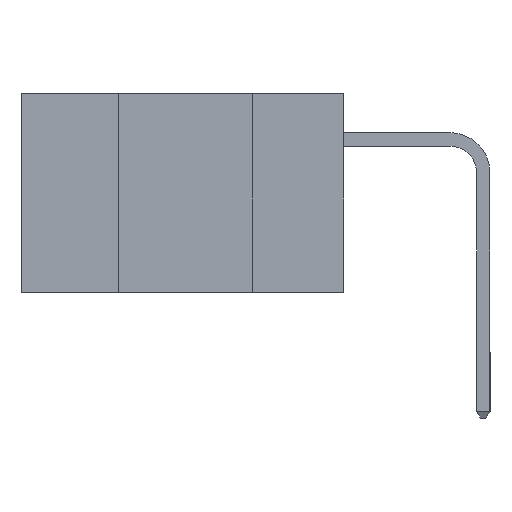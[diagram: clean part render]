
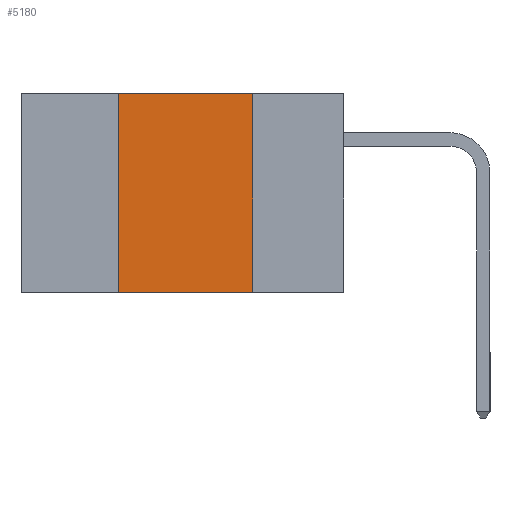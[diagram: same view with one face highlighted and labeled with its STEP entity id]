
A CAD part, left-side view. The second image highlights one B-rep face of the part: STEP entity #5180.
In plain terms, the highlighted planar face has unit normal (-1, 0, 0).
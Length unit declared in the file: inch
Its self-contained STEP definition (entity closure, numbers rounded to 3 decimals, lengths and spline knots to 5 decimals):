
#201 = EDGE_LOOP ( 'NONE', ( #4824, #17462, #16086, #9617 ) ) ;
#667 = EDGE_CURVE ( 'NONE', #13989, #11770, #18089, .T. ) ;
#1258 = VERTEX_POINT ( 'NONE', #18324 ) ;
#1557 = CARTESIAN_POINT ( 'NONE',  ( 0., 0.17, -0.37 ) ) ;
#1958 = CARTESIAN_POINT ( 'NONE',  ( 0., 0.6, -0.37 ) ) ;
#2879 = DIRECTION ( 'NONE',  ( 0., 0., 1. ) ) ;
#3065 = LINE ( 'NONE', #11438, #11336 ) ;
#3340 = LINE ( 'NONE', #1958, #9825 ) ;
#3474 = CARTESIAN_POINT ( 'NONE',  ( 0., 0.17, 0. ) ) ;
#4751 = AXIS2_PLACEMENT_3D ( 'NONE', #9427, #13725, #5181 ) ;
#4824 = ORIENTED_EDGE ( 'NONE', *, *, #667, .F. ) ;
#5180 = ADVANCED_FACE ( 'NONE', ( #17553 ), #12529, .F. ) ;
#5181 = DIRECTION ( 'NONE',  ( 0., 0., -1. ) ) ;
#6953 = LINE ( 'NONE', #16270, #18117 ) ;
#7706 = DIRECTION ( 'NONE',  ( 0., -1., 0. ) ) ;
#8925 = VECTOR ( 'NONE', #12486, 39.37008 ) ;
#8936 = EDGE_CURVE ( 'NONE', #18124, #13989, #6953, .T. ) ;
#9427 = CARTESIAN_POINT ( 'NONE',  ( 0., 0.6, 0. ) ) ;
#9617 = ORIENTED_EDGE ( 'NONE', *, *, #14558, .T. ) ;
#9825 = VECTOR ( 'NONE', #7706, 39.37008 ) ;
#11336 = VECTOR ( 'NONE', #2879, 39.37008 ) ;
#11438 = CARTESIAN_POINT ( 'NONE',  ( 0., 0.42, 0. ) ) ;
#11770 = VERTEX_POINT ( 'NONE', #1557 ) ;
#12486 = DIRECTION ( 'NONE',  ( 0., 0., -1. ) ) ;
#12529 = PLANE ( 'NONE',  #4751 ) ;
#13269 = DIRECTION ( 'NONE',  ( 0., -1., 0. ) ) ;
#13725 = DIRECTION ( 'NONE',  ( 1., 0., 0. ) ) ;
#13989 = VERTEX_POINT ( 'NONE', #3474 ) ;
#14558 = EDGE_CURVE ( 'NONE', #1258, #11770, #3340, .T. ) ;
#16086 = ORIENTED_EDGE ( 'NONE', *, *, #16196, .F. ) ;
#16196 = EDGE_CURVE ( 'NONE', #1258, #18124, #3065, .T. ) ;
#16270 = CARTESIAN_POINT ( 'NONE',  ( 0., 0.6, 0. ) ) ;
#16804 = CARTESIAN_POINT ( 'NONE',  ( 0., 0.17, 0. ) ) ;
#17199 = CARTESIAN_POINT ( 'NONE',  ( 0., 0.42, 0. ) ) ;
#17462 = ORIENTED_EDGE ( 'NONE', *, *, #8936, .F. ) ;
#17553 = FACE_OUTER_BOUND ( 'NONE', #201, .T. ) ;
#18089 = LINE ( 'NONE', #16804, #8925 ) ;
#18117 = VECTOR ( 'NONE', #13269, 39.37008 ) ;
#18124 = VERTEX_POINT ( 'NONE', #17199 ) ;
#18324 = CARTESIAN_POINT ( 'NONE',  ( 0., 0.42, -0.37 ) ) ;
